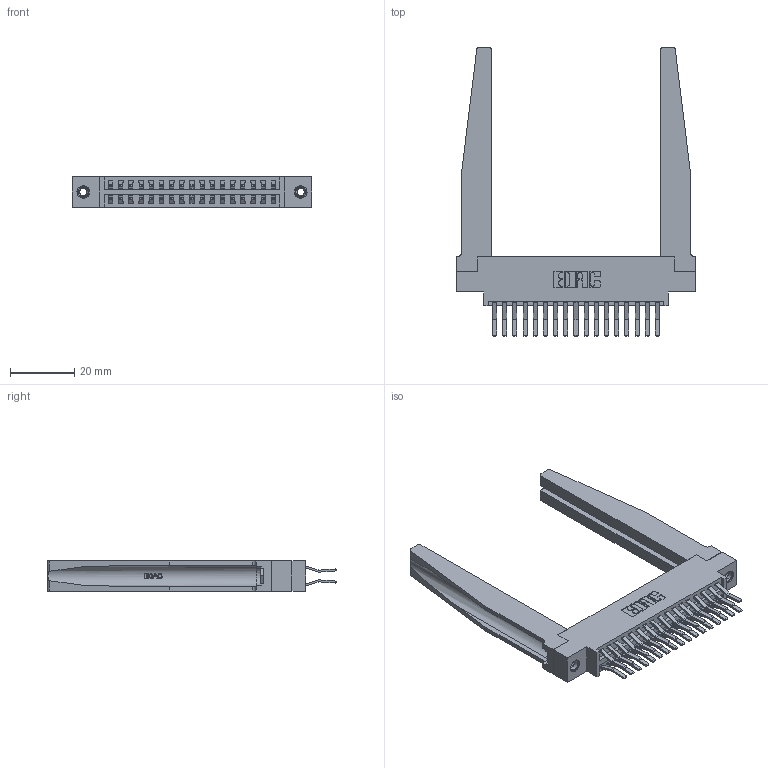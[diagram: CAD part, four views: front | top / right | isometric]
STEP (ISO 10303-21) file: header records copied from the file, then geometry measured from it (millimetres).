
FILE_DESCRIPTION (( 'STEP AP203' ), '1' );
FILE_NAME ('346-034-560-878.STEP', '2022-05-19T20:45:07', ( '' ), ( '' ), 'SwSTEP 2.0', 'SolidWorks 2020', '' );
FILE_SCHEMA (( 'CONFIG_CONTROL_DESIGN' ));
Length unit declared in the file: inch
Products named in the file (5): 346 Part_0.170 Offset - 0.156 Dia-TH; 345-250-001_345-250-001-102; 346-034-560-878; 345-292-001_560 Tail; 346-220-078_345-220-078
Assembly tree (39 placements, depth 2):
  346-034-560-878
    346 Part_0.170 Offset - 0.156 Dia-TH
    345-292-001_560 Tail  x34
    346-220-078_345-220-078  x2
    345-250-001_345-250-001-102  x2
Bounding box: 74.55 x 90.05 x 9.4 mm (x, y, z)
Volume: 14034.3 mm3; surface area: 16747.7 mm2
Topology: 39 solids, 39 shells, 2210 faces, 6459 edges, 4250 vertices
Faces by surface type: plane 1426, cylinder 732, bspline 36, cone 12, torus 4
Entity records: 19844 total; most frequent: CARTESIAN_POINT 4249, ORIENTED_EDGE 3070, DIRECTION 2785, EDGE_CURVE 1535, VECTOR 1237, LINE 1237, VERTEX_POINT 1016, AXIS2_PLACEMENT_3D 774
